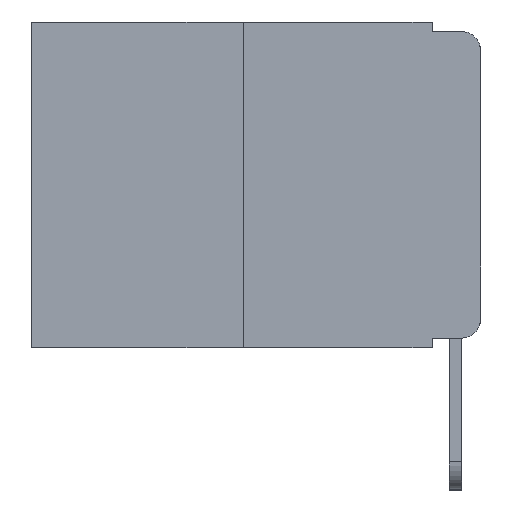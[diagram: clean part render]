
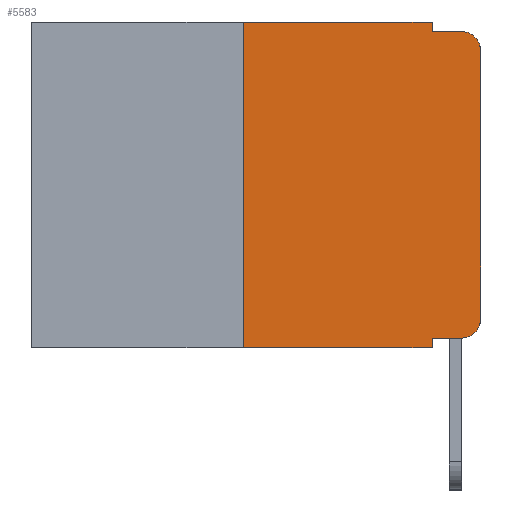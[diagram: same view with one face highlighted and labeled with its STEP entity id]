
A CAD part, left-side view. The second image highlights one B-rep face of the part: STEP entity #5583.
In plain terms, the highlighted planar face has unit normal (-1, 0, 0).
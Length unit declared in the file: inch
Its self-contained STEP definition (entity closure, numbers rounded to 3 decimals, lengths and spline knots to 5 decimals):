
#190 = DIRECTION ( 'NONE',  ( 0., -1., 0. ) ) ;
#613 = VERTEX_POINT ( 'NONE', #6227 ) ;
#791 = CARTESIAN_POINT ( 'NONE',  ( 0., 0.051, -0.01 ) ) ;
#964 = CARTESIAN_POINT ( 'NONE',  ( 0., 0.051, -0.01 ) ) ;
#1012 = ORIENTED_EDGE ( 'NONE', *, *, #4787, .F. ) ;
#1215 = CARTESIAN_POINT ( 'NONE',  ( 0., 0.051, 0. ) ) ;
#1335 = VERTEX_POINT ( 'NONE', #8402 ) ;
#1353 = DIRECTION ( 'NONE',  ( 0., 0., -1. ) ) ;
#1400 = CARTESIAN_POINT ( 'NONE',  ( 0., 0.473, -0.343 ) ) ;
#1451 = LINE ( 'NONE', #964, #3258 ) ;
#1503 = VECTOR ( 'NONE', #6284, 39.37008 ) ;
#1933 = DIRECTION ( 'NONE',  ( 0., 0., -1. ) ) ;
#1960 = DIRECTION ( 'NONE',  ( 0., 0., -1. ) ) ;
#2084 = ORIENTED_EDGE ( 'NONE', *, *, #7976, .T. ) ;
#2116 = DIRECTION ( 'NONE',  ( 0., -1., 0. ) ) ;
#2123 = LINE ( 'NONE', #4063, #5986 ) ;
#2227 = CARTESIAN_POINT ( 'NONE',  ( 0., 0.473, 0. ) ) ;
#2489 = ORIENTED_EDGE ( 'NONE', *, *, #6575, .F. ) ;
#2821 = FACE_OUTER_BOUND ( 'NONE', #5549, .T. ) ;
#3043 = LINE ( 'NONE', #2227, #5611 ) ;
#3258 = VECTOR ( 'NONE', #190, 39.37008 ) ;
#3269 = CARTESIAN_POINT ( 'NONE',  ( 0., 0.02, -0.333 ) ) ;
#3473 = ORIENTED_EDGE ( 'NONE', *, *, #10506, .F. ) ;
#3524 = VECTOR ( 'NONE', #4451, 39.37008 ) ;
#3563 = DIRECTION ( 'NONE',  ( 0., 0., -1. ) ) ;
#3566 = CARTESIAN_POINT ( 'NONE',  ( 0., 0.473, 0. ) ) ;
#3624 = VECTOR ( 'NONE', #2116, 39.37008 ) ;
#3787 = VERTEX_POINT ( 'NONE', #6858 ) ;
#3830 = LINE ( 'NONE', #1215, #9671 ) ;
#4063 = CARTESIAN_POINT ( 'NONE',  ( 0., 0.051, -0.333 ) ) ;
#4267 = AXIS2_PLACEMENT_3D ( 'NONE', #8439, #9178, #3563 ) ;
#4316 = AXIS2_PLACEMENT_3D ( 'NONE', #3566, #8503, #1933 ) ;
#4451 = DIRECTION ( 'NONE',  ( 0., 0., 1. ) ) ;
#4659 = VERTEX_POINT ( 'NONE', #7169 ) ;
#4699 = VERTEX_POINT ( 'NONE', #5197 ) ;
#4716 = CARTESIAN_POINT ( 'NONE',  ( 0., 0.051, -0.343 ) ) ;
#4787 = EDGE_CURVE ( 'NONE', #613, #6195, #5609, .T. ) ;
#5083 = CIRCLE ( 'NONE', #4267, 0.02 ) ;
#5156 = EDGE_CURVE ( 'NONE', #10125, #6609, #10219, .T. ) ;
#5197 = CARTESIAN_POINT ( 'NONE',  ( 0., 0., -0.313 ) ) ;
#5231 = CARTESIAN_POINT ( 'NONE',  ( 0., 0., 0. ) ) ;
#5273 = DIRECTION ( 'NONE',  ( -1., 0., 0. ) ) ;
#5472 = ORIENTED_EDGE ( 'NONE', *, *, #7215, .F. ) ;
#5535 = CARTESIAN_POINT ( 'NONE',  ( 0., 0.25, 0. ) ) ;
#5549 = EDGE_LOOP ( 'NONE', ( #9383, #2084, #3473, #1012, #5472, #7253, #7322, #2489, #9955, #6373 ) ) ;
#5583 = ADVANCED_FACE ( 'NONE', ( #2821 ), #8442, .F. ) ;
#5609 = LINE ( 'NONE', #7054, #1503 ) ;
#5611 = VECTOR ( 'NONE', #7907, 39.37008 ) ;
#5986 = VECTOR ( 'NONE', #10525, 39.37008 ) ;
#6090 = LINE ( 'NONE', #7378, #9268 ) ;
#6195 = VERTEX_POINT ( 'NONE', #791 ) ;
#6227 = CARTESIAN_POINT ( 'NONE',  ( 0., 0.051, 0. ) ) ;
#6284 = DIRECTION ( 'NONE',  ( 0., 0., -1. ) ) ;
#6373 = ORIENTED_EDGE ( 'NONE', *, *, #6407, .T. ) ;
#6407 = EDGE_CURVE ( 'NONE', #9491, #4699, #8416, .T. ) ;
#6489 = DIRECTION ( 'NONE',  ( 0., 0., 1. ) ) ;
#6575 = EDGE_CURVE ( 'NONE', #1335, #6609, #3830, .T. ) ;
#6609 = VERTEX_POINT ( 'NONE', #4716 ) ;
#6826 = LINE ( 'NONE', #5231, #3524 ) ;
#6858 = CARTESIAN_POINT ( 'NONE',  ( 0., 0., -0.03 ) ) ;
#7054 = CARTESIAN_POINT ( 'NONE',  ( 0., 0.051, 0. ) ) ;
#7169 = CARTESIAN_POINT ( 'NONE',  ( 0., 0.02, -0.01 ) ) ;
#7215 = EDGE_CURVE ( 'NONE', #7720, #613, #3043, .T. ) ;
#7253 = ORIENTED_EDGE ( 'NONE', *, *, #7626, .F. ) ;
#7322 = ORIENTED_EDGE ( 'NONE', *, *, #5156, .T. ) ;
#7378 = CARTESIAN_POINT ( 'NONE',  ( 0., 0.25, 0. ) ) ;
#7626 = EDGE_CURVE ( 'NONE', #10125, #7720, #6090, .T. ) ;
#7720 = VERTEX_POINT ( 'NONE', #5535 ) ;
#7907 = DIRECTION ( 'NONE',  ( 0., -1., 0. ) ) ;
#7976 = EDGE_CURVE ( 'NONE', #3787, #4659, #5083, .T. ) ;
#8402 = CARTESIAN_POINT ( 'NONE',  ( 0., 0.051, -0.333 ) ) ;
#8416 = CIRCLE ( 'NONE', #9336, 0.02 ) ;
#8439 = CARTESIAN_POINT ( 'NONE',  ( 0., 0.02, -0.03 ) ) ;
#8442 = PLANE ( 'NONE',  #4316 ) ;
#8503 = DIRECTION ( 'NONE',  ( 1., 0., 0. ) ) ;
#9021 = CARTESIAN_POINT ( 'NONE',  ( 0., 0.25, -0.343 ) ) ;
#9178 = DIRECTION ( 'NONE',  ( -1., 0., 0. ) ) ;
#9211 = CARTESIAN_POINT ( 'NONE',  ( 0., 0.02, -0.313 ) ) ;
#9268 = VECTOR ( 'NONE', #6489, 39.37008 ) ;
#9336 = AXIS2_PLACEMENT_3D ( 'NONE', #9211, #5273, #1960 ) ;
#9383 = ORIENTED_EDGE ( 'NONE', *, *, #10544, .T. ) ;
#9491 = VERTEX_POINT ( 'NONE', #3269 ) ;
#9511 = EDGE_CURVE ( 'NONE', #1335, #9491, #2123, .T. ) ;
#9671 = VECTOR ( 'NONE', #1353, 39.37008 ) ;
#9955 = ORIENTED_EDGE ( 'NONE', *, *, #9511, .T. ) ;
#10125 = VERTEX_POINT ( 'NONE', #9021 ) ;
#10219 = LINE ( 'NONE', #1400, #3624 ) ;
#10506 = EDGE_CURVE ( 'NONE', #6195, #4659, #1451, .T. ) ;
#10525 = DIRECTION ( 'NONE',  ( 0., -1., 0. ) ) ;
#10544 = EDGE_CURVE ( 'NONE', #4699, #3787, #6826, .T. ) ;
